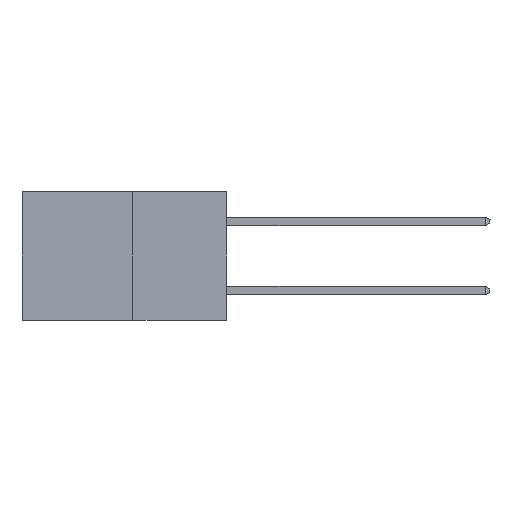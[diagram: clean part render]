
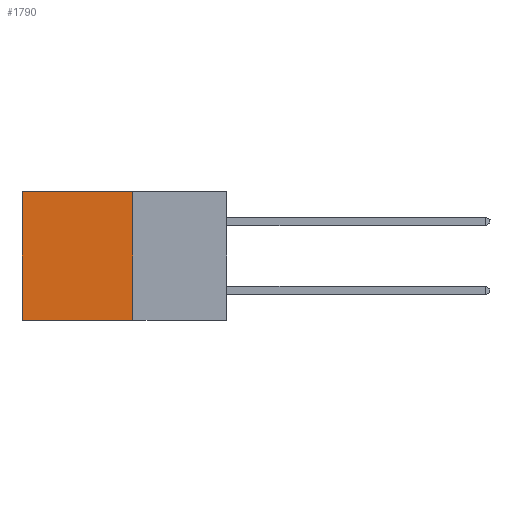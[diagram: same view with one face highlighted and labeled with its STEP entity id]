
A CAD part, left-side view. The second image highlights one B-rep face of the part: STEP entity #1790.
In plain terms, the highlighted planar face has unit normal (-1, 0, 0).
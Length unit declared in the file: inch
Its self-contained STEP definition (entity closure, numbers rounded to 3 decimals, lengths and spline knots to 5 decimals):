
#654 = EDGE_CURVE ( 'NONE', #5633, #7442, #8544, .T. ) ;
#847 = DIRECTION ( 'NONE',  ( 0., 0., -1. ) ) ;
#938 = ORIENTED_EDGE ( 'NONE', *, *, #7302, .T. ) ;
#956 = PLANE ( 'NONE',  #5190 ) ;
#971 = DIRECTION ( 'NONE',  ( 0., 1., 0. ) ) ;
#1192 = DIRECTION ( 'NONE',  ( 0., 0., -1. ) ) ;
#1240 = CARTESIAN_POINT ( 'NONE',  ( 0.277, 0.27, 0. ) ) ;
#1267 = CARTESIAN_POINT ( 'NONE',  ( 0.277, 0.27, 0. ) ) ;
#1790 = ADVANCED_FACE ( 'NONE', ( #6399 ), #956, .F. ) ;
#1974 = DIRECTION ( 'NONE',  ( 1., 0., 0. ) ) ;
#2391 = CARTESIAN_POINT ( 'NONE',  ( 0.277, 0.27, -0.37 ) ) ;
#2635 = EDGE_CURVE ( 'NONE', #3837, #5633, #6074, .T. ) ;
#2701 = CARTESIAN_POINT ( 'NONE',  ( 0.277, 0.27, -0.37 ) ) ;
#2774 = DIRECTION ( 'NONE',  ( 0., 0., -1. ) ) ;
#2937 = CARTESIAN_POINT ( 'NONE',  ( 0.277, 0.27, -0.37 ) ) ;
#3539 = CARTESIAN_POINT ( 'NONE',  ( 0.277, 0.59, -0.37 ) ) ;
#3837 = VERTEX_POINT ( 'NONE', #1240 ) ;
#4017 = EDGE_CURVE ( 'NONE', #4485, #7442, #6347, .T. ) ;
#4124 = ORIENTED_EDGE ( 'NONE', *, *, #4017, .T. ) ;
#4213 = VECTOR ( 'NONE', #847, 39.37008 ) ;
#4485 = VERTEX_POINT ( 'NONE', #4590 ) ;
#4590 = CARTESIAN_POINT ( 'NONE',  ( 0.277, 0.59, 0. ) ) ;
#4649 = LINE ( 'NONE', #1267, #8330 ) ;
#5190 = AXIS2_PLACEMENT_3D ( 'NONE', #2701, #1974, #1192 ) ;
#5633 = VERTEX_POINT ( 'NONE', #6127 ) ;
#6074 = LINE ( 'NONE', #2937, #4213 ) ;
#6127 = CARTESIAN_POINT ( 'NONE',  ( 0.277, 0.27, -0.37 ) ) ;
#6191 = ORIENTED_EDGE ( 'NONE', *, *, #654, .F. ) ;
#6347 = LINE ( 'NONE', #3539, #7777 ) ;
#6399 = FACE_OUTER_BOUND ( 'NONE', #6912, .T. ) ;
#6912 = EDGE_LOOP ( 'NONE', ( #4124, #6191, #7820, #938 ) ) ;
#7302 = EDGE_CURVE ( 'NONE', #3837, #4485, #4649, .T. ) ;
#7442 = VERTEX_POINT ( 'NONE', #7764 ) ;
#7764 = CARTESIAN_POINT ( 'NONE',  ( 0.277, 0.59, -0.37 ) ) ;
#7777 = VECTOR ( 'NONE', #2774, 39.37008 ) ;
#7820 = ORIENTED_EDGE ( 'NONE', *, *, #2635, .F. ) ;
#8330 = VECTOR ( 'NONE', #971, 39.37008 ) ;
#8340 = DIRECTION ( 'NONE',  ( 0., 1., 0. ) ) ;
#8359 = VECTOR ( 'NONE', #8340, 39.37008 ) ;
#8544 = LINE ( 'NONE', #2391, #8359 ) ;
